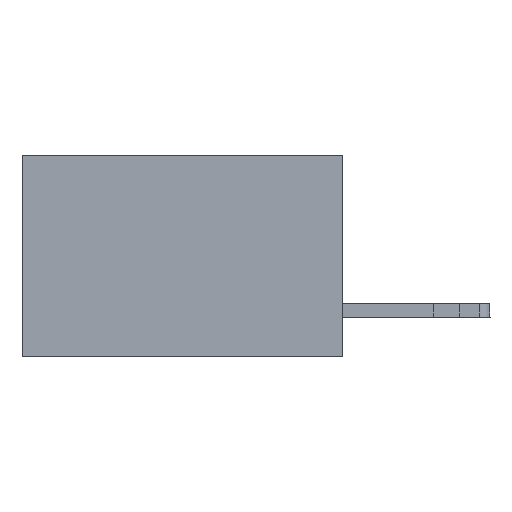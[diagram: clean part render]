
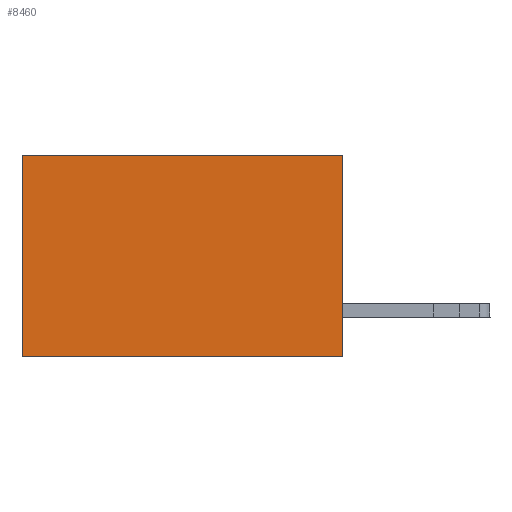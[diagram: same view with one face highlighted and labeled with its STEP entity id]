
A CAD part, left-side view. The second image highlights one B-rep face of the part: STEP entity #8460.
In plain terms, the highlighted planar face has unit normal (-1, 0, 0).
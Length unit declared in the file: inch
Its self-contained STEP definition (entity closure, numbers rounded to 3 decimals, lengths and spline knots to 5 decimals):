
#240 = EDGE_CURVE ( 'NONE', #8226, #8116, #1977, .T. ) ;
#247 = PLANE ( 'NONE',  #10624 ) ;
#323 = VERTEX_POINT ( 'NONE', #4922 ) ;
#1488 = CARTESIAN_POINT ( 'NONE',  ( 0.277, 0., -0.37 ) ) ;
#1543 = LINE ( 'NONE', #10065, #7748 ) ;
#1977 = LINE ( 'NONE', #8332, #2355 ) ;
#2355 = VECTOR ( 'NONE', #5009, 39.37008 ) ;
#2723 = DIRECTION ( 'NONE',  ( 1., 0., 0. ) ) ;
#4314 = VECTOR ( 'NONE', #14828, 39.37008 ) ;
#4922 = CARTESIAN_POINT ( 'NONE',  ( 0.277, 0.59, -0.37 ) ) ;
#5009 = DIRECTION ( 'NONE',  ( 0., 1., 0. ) ) ;
#5163 = CARTESIAN_POINT ( 'NONE',  ( 0.277, 0., -0.37 ) ) ;
#5243 = CARTESIAN_POINT ( 'NONE',  ( 0.277, 0., -0.37 ) ) ;
#5807 = EDGE_CURVE ( 'NONE', #8116, #323, #13282, .T. ) ;
#6325 = ORIENTED_EDGE ( 'NONE', *, *, #5807, .T. ) ;
#6707 = VECTOR ( 'NONE', #12560, 39.37008 ) ;
#7077 = VERTEX_POINT ( 'NONE', #5163 ) ;
#7364 = FACE_OUTER_BOUND ( 'NONE', #8810, .T. ) ;
#7748 = VECTOR ( 'NONE', #11242, 39.37008 ) ;
#8116 = VERTEX_POINT ( 'NONE', #11786 ) ;
#8226 = VERTEX_POINT ( 'NONE', #12097 ) ;
#8332 = CARTESIAN_POINT ( 'NONE',  ( 0.277, 0., 0. ) ) ;
#8401 = EDGE_CURVE ( 'NONE', #7077, #323, #1543, .T. ) ;
#8460 = ADVANCED_FACE ( 'NONE', ( #7364 ), #247, .F. ) ;
#8810 = EDGE_LOOP ( 'NONE', ( #6325, #8942, #10920, #11300 ) ) ;
#8942 = ORIENTED_EDGE ( 'NONE', *, *, #8401, .F. ) ;
#10065 = CARTESIAN_POINT ( 'NONE',  ( 0.277, 0., -0.37 ) ) ;
#10624 = AXIS2_PLACEMENT_3D ( 'NONE', #1488, #2723, #11342 ) ;
#10920 = ORIENTED_EDGE ( 'NONE', *, *, #11154, .F. ) ;
#11154 = EDGE_CURVE ( 'NONE', #8226, #7077, #13526, .T. ) ;
#11242 = DIRECTION ( 'NONE',  ( 0., 1., 0. ) ) ;
#11300 = ORIENTED_EDGE ( 'NONE', *, *, #240, .T. ) ;
#11342 = DIRECTION ( 'NONE',  ( 0., 0., -1. ) ) ;
#11786 = CARTESIAN_POINT ( 'NONE',  ( 0.277, 0.59, 0. ) ) ;
#12097 = CARTESIAN_POINT ( 'NONE',  ( 0.277, 0., 0. ) ) ;
#12560 = DIRECTION ( 'NONE',  ( 0., 0., -1. ) ) ;
#13282 = LINE ( 'NONE', #15224, #4314 ) ;
#13526 = LINE ( 'NONE', #5243, #6707 ) ;
#14828 = DIRECTION ( 'NONE',  ( 0., 0., -1. ) ) ;
#15224 = CARTESIAN_POINT ( 'NONE',  ( 0.277, 0.59, -0.37 ) ) ;
